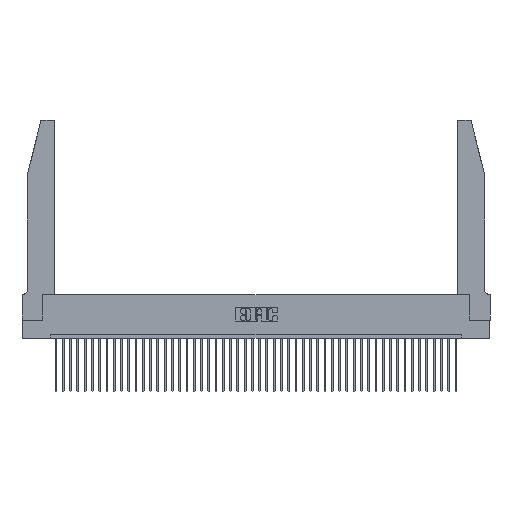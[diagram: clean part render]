
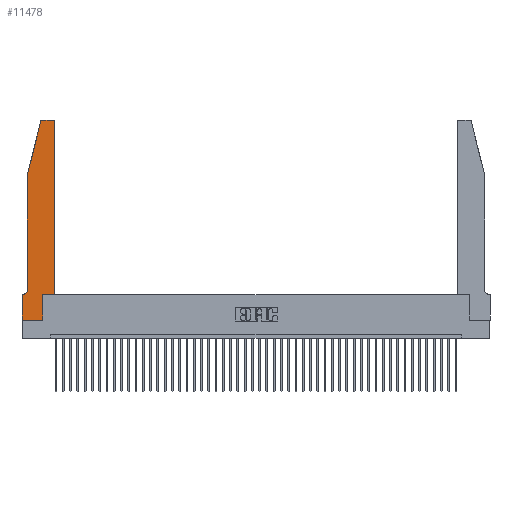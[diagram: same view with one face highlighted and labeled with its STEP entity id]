
A CAD part, top view. The second image highlights one B-rep face of the part: STEP entity #11478.
In plain terms, the highlighted planar face has unit normal (0, 0, 1).
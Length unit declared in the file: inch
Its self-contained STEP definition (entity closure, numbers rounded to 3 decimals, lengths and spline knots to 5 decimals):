
#2661 = ORIENTED_EDGE ( 'NONE', *, *, #34480, .T. ) ;
#3603 = EDGE_CURVE ( 'NONE', #9004, #38001, #25414, .T. ) ;
#3918 = VECTOR ( 'NONE', #25205, 39.37008 ) ;
#3949 = LINE ( 'NONE', #26427, #35025 ) ;
#4319 = CARTESIAN_POINT ( 'NONE',  ( 0., 0., 0.37 ) ) ;
#4639 = EDGE_LOOP ( 'NONE', ( #27484, #40246, #9366, #15195, #41804, #2661, #10595, #10556, #34947, #42527, #31652, #31876 ) ) ;
#6556 = CARTESIAN_POINT ( 'NONE',  ( 0.284, 2.75, 0.37 ) ) ;
#6608 = AXIS2_PLACEMENT_3D ( 'NONE', #16315, #37009, #33833 ) ;
#9004 = VERTEX_POINT ( 'NONE', #21204 ) ;
#9366 = ORIENTED_EDGE ( 'NONE', *, *, #37527, .T. ) ;
#9792 = DIRECTION ( 'NONE',  ( 0., -1., 0. ) ) ;
#10300 = VECTOR ( 'NONE', #30127, 39.37008 ) ;
#10556 = ORIENTED_EDGE ( 'NONE', *, *, #24583, .T. ) ;
#10595 = ORIENTED_EDGE ( 'NONE', *, *, #43602, .T. ) ;
#10887 = EDGE_CURVE ( 'NONE', #23443, #17685, #3949, .T. ) ;
#11165 = DIRECTION ( 'NONE',  ( -1., 0., 0. ) ) ;
#11478 = ADVANCED_FACE ( 'NONE', ( #44180 ), #19800, .T. ) ;
#11870 = VERTEX_POINT ( 'NONE', #44585 ) ;
#12682 = CARTESIAN_POINT ( 'NONE',  ( 0.2865, 0., 0.37 ) ) ;
#13311 = AXIS2_PLACEMENT_3D ( 'NONE', #28695, #36138, #43232 ) ;
#13810 = EDGE_CURVE ( 'NONE', #33907, #39563, #28812, .T. ) ;
#14276 = VERTEX_POINT ( 'NONE', #36386 ) ;
#14783 = CARTESIAN_POINT ( 'NONE',  ( 0.0055, 0.42, 0.37 ) ) ;
#15195 = ORIENTED_EDGE ( 'NONE', *, *, #28123, .T. ) ;
#15289 = CARTESIAN_POINT ( 'NONE',  ( 0.4505, 2.72, 0.37 ) ) ;
#16156 = LINE ( 'NONE', #26901, #33603 ) ;
#16315 = CARTESIAN_POINT ( 'NONE',  ( 0., 0.35, 0.37 ) ) ;
#16848 = VERTEX_POINT ( 'NONE', #32431 ) ;
#17685 = VERTEX_POINT ( 'NONE', #6556 ) ;
#17741 = CIRCLE ( 'NONE', #13311, 0.03 ) ;
#19134 = EDGE_CURVE ( 'NONE', #17685, #29651, #22505, .T. ) ;
#19514 = EDGE_CURVE ( 'NONE', #35479, #14276, #24672, .T. ) ;
#19799 = LINE ( 'NONE', #35254, #26922 ) ;
#19800 = PLANE ( 'NONE',  #6608 ) ;
#20076 = LINE ( 'NONE', #44378, #43993 ) ;
#21204 = CARTESIAN_POINT ( 'NONE',  ( 0.4505, 0.35, 0.37 ) ) ;
#21721 = VECTOR ( 'NONE', #34705, 39.37008 ) ;
#22505 = CIRCLE ( 'NONE', #44109, 0.03 ) ;
#23188 = CARTESIAN_POINT ( 'NONE',  ( 0., 0., 0.37 ) ) ;
#23443 = VERTEX_POINT ( 'NONE', #40188 ) ;
#23829 = VECTOR ( 'NONE', #9792, 39.37008 ) ;
#23933 = AXIS2_PLACEMENT_3D ( 'NONE', #14783, #35924, #11165 ) ;
#24271 = DIRECTION ( 'NONE',  ( 0., 1., 0. ) ) ;
#24583 = EDGE_CURVE ( 'NONE', #29692, #35479, #40225, .T. ) ;
#24672 = LINE ( 'NONE', #31905, #3918 ) ;
#25205 = DIRECTION ( 'NONE',  ( 0., 1., 0. ) ) ;
#25414 = LINE ( 'NONE', #31537, #31964 ) ;
#26396 = DIRECTION ( 'NONE',  ( 0., 0., 1. ) ) ;
#26427 = CARTESIAN_POINT ( 'NONE',  ( 0.2605, 2.75, 0.37 ) ) ;
#26901 = CARTESIAN_POINT ( 'NONE',  ( 0.0755, 2., 0.37 ) ) ;
#26922 = VECTOR ( 'NONE', #38276, 39.37008 ) ;
#27484 = ORIENTED_EDGE ( 'NONE', *, *, #10887, .T. ) ;
#28123 = EDGE_CURVE ( 'NONE', #11870, #33907, #16156, .T. ) ;
#28313 = LINE ( 'NONE', #36500, #10300 ) ;
#28695 = CARTESIAN_POINT ( 'NONE',  ( 0.4205, 2.72, 0.37 ) ) ;
#28812 = CIRCLE ( 'NONE', #23933, 0.07 ) ;
#29651 = VERTEX_POINT ( 'NONE', #36187 ) ;
#29692 = VERTEX_POINT ( 'NONE', #4319 ) ;
#30127 = DIRECTION ( 'NONE',  ( 1., 0., 0. ) ) ;
#30758 = DIRECTION ( 'NONE',  ( -0.239, -0.971, 0. ) ) ;
#31537 = CARTESIAN_POINT ( 'NONE',  ( 0.4505, 0.35, 0.37 ) ) ;
#31652 = ORIENTED_EDGE ( 'NONE', *, *, #3603, .T. ) ;
#31795 = CARTESIAN_POINT ( 'NONE',  ( 0.0755, 0.42, 0.37 ) ) ;
#31876 = ORIENTED_EDGE ( 'NONE', *, *, #44003, .T. ) ;
#31905 = CARTESIAN_POINT ( 'NONE',  ( 0.2865, 0.35, 0.37 ) ) ;
#31964 = VECTOR ( 'NONE', #24271, 39.37008 ) ;
#32431 = CARTESIAN_POINT ( 'NONE',  ( 0., 0.35, 0.37 ) ) ;
#33603 = VECTOR ( 'NONE', #40805, 39.37008 ) ;
#33833 = DIRECTION ( 'NONE',  ( 1., 0., 0. ) ) ;
#33907 = VERTEX_POINT ( 'NONE', #31795 ) ;
#34480 = EDGE_CURVE ( 'NONE', #39563, #16848, #19799, .T. ) ;
#34705 = DIRECTION ( 'NONE',  ( 1., 0., 0. ) ) ;
#34947 = ORIENTED_EDGE ( 'NONE', *, *, #19514, .T. ) ;
#35025 = VECTOR ( 'NONE', #40198, 39.37008 ) ;
#35254 = CARTESIAN_POINT ( 'NONE',  ( 0.0755, 0.35, 0.37 ) ) ;
#35374 = CARTESIAN_POINT ( 'NONE',  ( 0.0055, 0.35, 0.37 ) ) ;
#35479 = VERTEX_POINT ( 'NONE', #12682 ) ;
#35924 = DIRECTION ( 'NONE',  ( 0., 0., -1. ) ) ;
#36138 = DIRECTION ( 'NONE',  ( 0., 0., 1. ) ) ;
#36187 = CARTESIAN_POINT ( 'NONE',  ( 0.25487, 2.72718, 0.37 ) ) ;
#36294 = LINE ( 'NONE', #23188, #23829 ) ;
#36386 = CARTESIAN_POINT ( 'NONE',  ( 0.2865, 0.35, 0.37 ) ) ;
#36500 = CARTESIAN_POINT ( 'NONE',  ( 0.4505, 0.35, 0.37 ) ) ;
#37009 = DIRECTION ( 'NONE',  ( 0., 0., 1. ) ) ;
#37527 = EDGE_CURVE ( 'NONE', #29651, #11870, #20076, .T. ) ;
#37600 = CARTESIAN_POINT ( 'NONE',  ( 0., 0., 0.37 ) ) ;
#38001 = VERTEX_POINT ( 'NONE', #15289 ) ;
#38276 = DIRECTION ( 'NONE',  ( -1., 0., 0. ) ) ;
#39085 = EDGE_CURVE ( 'NONE', #14276, #9004, #28313, .T. ) ;
#39563 = VERTEX_POINT ( 'NONE', #35374 ) ;
#40188 = CARTESIAN_POINT ( 'NONE',  ( 0.4205, 2.75, 0.37 ) ) ;
#40198 = DIRECTION ( 'NONE',  ( -1., 0., 0. ) ) ;
#40225 = LINE ( 'NONE', #37600, #21721 ) ;
#40246 = ORIENTED_EDGE ( 'NONE', *, *, #19134, .T. ) ;
#40805 = DIRECTION ( 'NONE',  ( 0., -1., 0. ) ) ;
#41804 = ORIENTED_EDGE ( 'NONE', *, *, #13810, .T. ) ;
#42527 = ORIENTED_EDGE ( 'NONE', *, *, #39085, .T. ) ;
#43232 = DIRECTION ( 'NONE',  ( 1., 0., 0. ) ) ;
#43602 = EDGE_CURVE ( 'NONE', #16848, #29692, #36294, .T. ) ;
#43661 = DIRECTION ( 'NONE',  ( 1., 0., 0. ) ) ;
#43993 = VECTOR ( 'NONE', #30758, 39.37008 ) ;
#44003 = EDGE_CURVE ( 'NONE', #38001, #23443, #17741, .T. ) ;
#44109 = AXIS2_PLACEMENT_3D ( 'NONE', #44122, #26396, #43661 ) ;
#44122 = CARTESIAN_POINT ( 'NONE',  ( 0.284, 2.72, 0.37 ) ) ;
#44180 = FACE_OUTER_BOUND ( 'NONE', #4639, .T. ) ;
#44378 = CARTESIAN_POINT ( 'NONE',  ( 0.0755, 2., 0.37 ) ) ;
#44585 = CARTESIAN_POINT ( 'NONE',  ( 0.0755, 2., 0.37 ) ) ;
